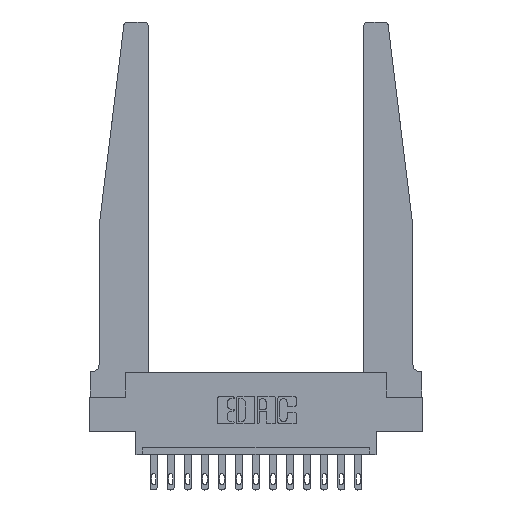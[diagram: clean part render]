
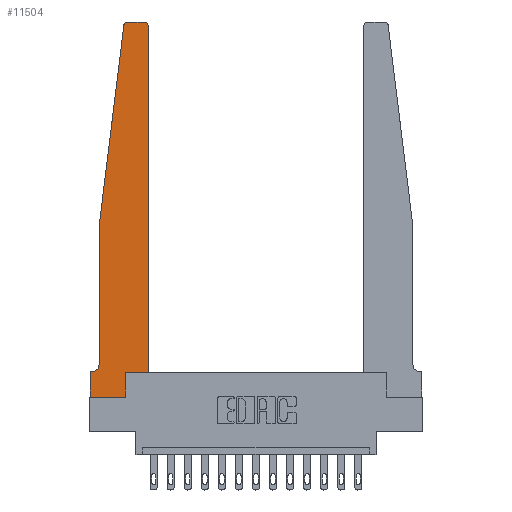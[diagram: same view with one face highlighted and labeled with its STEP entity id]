
A CAD part, top view. The second image highlights one B-rep face of the part: STEP entity #11504.
In plain terms, the highlighted planar face has unit normal (0, 0, 1).
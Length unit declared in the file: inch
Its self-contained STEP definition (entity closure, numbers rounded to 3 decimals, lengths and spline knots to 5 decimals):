
#85 = ORIENTED_EDGE ( 'NONE', *, *, #14203, .T. ) ;
#145 = AXIS2_PLACEMENT_3D ( 'NONE', #423, #7036, #6949 ) ;
#175 = CARTESIAN_POINT ( 'NONE',  ( 0.2605, 0., 0.37 ) ) ;
#423 = CARTESIAN_POINT ( 'NONE',  ( 0.395, 2.72, 0.37 ) ) ;
#473 = DIRECTION ( 'NONE',  ( -1., 0., 0. ) ) ;
#616 = AXIS2_PLACEMENT_3D ( 'NONE', #3049, #8361, #13669 ) ;
#685 = AXIS2_PLACEMENT_3D ( 'NONE', #10924, #15071, #6971 ) ;
#771 = VERTEX_POINT ( 'NONE', #175 ) ;
#1100 = CARTESIAN_POINT ( 'NONE',  ( 0., 0., 0.37 ) ) ;
#1101 = DIRECTION ( 'NONE',  ( 0., 1., 0. ) ) ;
#1122 = DIRECTION ( 'NONE',  ( 0., 0., 1. ) ) ;
#1302 = EDGE_CURVE ( 'NONE', #15732, #11408, #9125, .T. ) ;
#1695 = DIRECTION ( 'NONE',  ( 0., 1., 0. ) ) ;
#1718 = ORIENTED_EDGE ( 'NONE', *, *, #15096, .T. ) ;
#1753 = FACE_OUTER_BOUND ( 'NONE', #12169, .T. ) ;
#2190 = VERTEX_POINT ( 'NONE', #6112 ) ;
#2612 = VERTEX_POINT ( 'NONE', #16563 ) ;
#2880 = EDGE_CURVE ( 'NONE', #2612, #6151, #5559, .T. ) ;
#2933 = CIRCLE ( 'NONE', #145, 0.03 ) ;
#3001 = CARTESIAN_POINT ( 'NONE',  ( 0.24675, 2.72367, 0.37 ) ) ;
#3049 = CARTESIAN_POINT ( 'NONE',  ( 0.015, 0.2375, 0.37 ) ) ;
#3101 = VERTEX_POINT ( 'NONE', #17147 ) ;
#3812 = DIRECTION ( 'NONE',  ( 0., -1., 0. ) ) ;
#3958 = ORIENTED_EDGE ( 'NONE', *, *, #2880, .T. ) ;
#4111 = VERTEX_POINT ( 'NONE', #5738 ) ;
#4296 = EDGE_CURVE ( 'NONE', #4111, #2190, #6340, .T. ) ;
#4434 = ORIENTED_EDGE ( 'NONE', *, *, #4815, .T. ) ;
#4511 = LINE ( 'NONE', #15226, #11568 ) ;
#4791 = CARTESIAN_POINT ( 'NONE',  ( 0.065, 1.25, 0.37 ) ) ;
#4815 = EDGE_CURVE ( 'NONE', #771, #12473, #13539, .T. ) ;
#5033 = CARTESIAN_POINT ( 'NONE',  ( 0.25, 2.75, 0.37 ) ) ;
#5289 = DIRECTION ( 'NONE',  ( -1., 0., 0. ) ) ;
#5357 = VERTEX_POINT ( 'NONE', #11639 ) ;
#5559 = LINE ( 'NONE', #16190, #6957 ) ;
#5592 = ORIENTED_EDGE ( 'NONE', *, *, #10741, .T. ) ;
#5650 = ORIENTED_EDGE ( 'NONE', *, *, #10517, .T. ) ;
#5738 = CARTESIAN_POINT ( 'NONE',  ( 0.395, 2.75, 0.37 ) ) ;
#6112 = CARTESIAN_POINT ( 'NONE',  ( 0.27653, 2.75, 0.37 ) ) ;
#6151 = VERTEX_POINT ( 'NONE', #17052 ) ;
#6340 = LINE ( 'NONE', #5033, #9158 ) ;
#6438 = DIRECTION ( 'NONE',  ( 1., 0., 0. ) ) ;
#6949 = DIRECTION ( 'NONE',  ( 1., 0., 0. ) ) ;
#6957 = VECTOR ( 'NONE', #12281, 39.37008 ) ;
#6971 = DIRECTION ( 'NONE',  ( 1., 0., 0. ) ) ;
#7003 = CARTESIAN_POINT ( 'NONE',  ( 0.2605, 0.18, 0.37 ) ) ;
#7008 = VECTOR ( 'NONE', #8974, 39.37008 ) ;
#7036 = DIRECTION ( 'NONE',  ( 0., 0., 1. ) ) ;
#7101 = VECTOR ( 'NONE', #473, 39.37008 ) ;
#7243 = ORIENTED_EDGE ( 'NONE', *, *, #8832, .T. ) ;
#7322 = VECTOR ( 'NONE', #1101, 39.37008 ) ;
#7410 = CIRCLE ( 'NONE', #17164, 0.03 ) ;
#7605 = ORIENTED_EDGE ( 'NONE', *, *, #1302, .T. ) ;
#7744 = LINE ( 'NONE', #4791, #7008 ) ;
#8196 = VECTOR ( 'NONE', #3812, 39.37008 ) ;
#8361 = DIRECTION ( 'NONE',  ( 0., 0., -1. ) ) ;
#8695 = ORIENTED_EDGE ( 'NONE', *, *, #4296, .T. ) ;
#8832 = EDGE_CURVE ( 'NONE', #6151, #3101, #10650, .T. ) ;
#8894 = EDGE_CURVE ( 'NONE', #11261, #2612, #7744, .T. ) ;
#8974 = DIRECTION ( 'NONE',  ( -0.122, -0.992, 0. ) ) ;
#9125 = LINE ( 'NONE', #1100, #8196 ) ;
#9158 = VECTOR ( 'NONE', #5289, 39.37008 ) ;
#9843 = VECTOR ( 'NONE', #12177, 39.37008 ) ;
#9886 = CARTESIAN_POINT ( 'NONE',  ( 0.065, 0.1875, 0.37 ) ) ;
#10517 = EDGE_CURVE ( 'NONE', #5357, #16616, #14339, .T. ) ;
#10575 = CARTESIAN_POINT ( 'NONE',  ( 0., 0., 0.37 ) ) ;
#10650 = CIRCLE ( 'NONE', #616, 0.05 ) ;
#10741 = EDGE_CURVE ( 'NONE', #11408, #771, #13214, .T. ) ;
#10924 = CARTESIAN_POINT ( 'NONE',  ( 0., 0.1875, 0.37 ) ) ;
#11150 = CARTESIAN_POINT ( 'NONE',  ( 0.425, 2.72, 0.37 ) ) ;
#11184 = PLANE ( 'NONE',  #685 ) ;
#11261 = VERTEX_POINT ( 'NONE', #3001 ) ;
#11408 = VERTEX_POINT ( 'NONE', #10575 ) ;
#11504 = ADVANCED_FACE ( 'NONE', ( #1753 ), #11184, .T. ) ;
#11568 = VECTOR ( 'NONE', #13663, 39.37008 ) ;
#11639 = CARTESIAN_POINT ( 'NONE',  ( 0.425, 0.18, 0.37 ) ) ;
#11848 = CARTESIAN_POINT ( 'NONE',  ( 0., 0.1875, 0.37 ) ) ;
#12169 = EDGE_LOOP ( 'NONE', ( #8695, #15881, #12314, #3958, #7243, #1718, #7605, #5592, #4434, #13002, #5650, #85 ) ) ;
#12177 = DIRECTION ( 'NONE',  ( 1., 0., 0. ) ) ;
#12281 = DIRECTION ( 'NONE',  ( 0., -1., 0. ) ) ;
#12314 = ORIENTED_EDGE ( 'NONE', *, *, #8894, .T. ) ;
#12408 = LINE ( 'NONE', #9886, #7101 ) ;
#12473 = VERTEX_POINT ( 'NONE', #15520 ) ;
#13002 = ORIENTED_EDGE ( 'NONE', *, *, #14178, .T. ) ;
#13056 = CARTESIAN_POINT ( 'NONE',  ( 0.27653, 2.72, 0.37 ) ) ;
#13214 = LINE ( 'NONE', #16081, #9843 ) ;
#13539 = LINE ( 'NONE', #7003, #16159 ) ;
#13663 = DIRECTION ( 'NONE',  ( 1., 0., 0. ) ) ;
#13669 = DIRECTION ( 'NONE',  ( -1., 0., 0. ) ) ;
#14165 = CARTESIAN_POINT ( 'NONE',  ( 0.425, 0.18, 0.37 ) ) ;
#14178 = EDGE_CURVE ( 'NONE', #12473, #5357, #4511, .T. ) ;
#14203 = EDGE_CURVE ( 'NONE', #16616, #4111, #2933, .T. ) ;
#14339 = LINE ( 'NONE', #14165, #7322 ) ;
#15071 = DIRECTION ( 'NONE',  ( 0., 0., 1. ) ) ;
#15096 = EDGE_CURVE ( 'NONE', #3101, #15732, #12408, .T. ) ;
#15226 = CARTESIAN_POINT ( 'NONE',  ( 0.425, 0.18, 0.37 ) ) ;
#15520 = CARTESIAN_POINT ( 'NONE',  ( 0.2605, 0.18, 0.37 ) ) ;
#15732 = VERTEX_POINT ( 'NONE', #11848 ) ;
#15881 = ORIENTED_EDGE ( 'NONE', *, *, #16460, .T. ) ;
#16081 = CARTESIAN_POINT ( 'NONE',  ( 0., 0., 0.37 ) ) ;
#16159 = VECTOR ( 'NONE', #1695, 39.37008 ) ;
#16190 = CARTESIAN_POINT ( 'NONE',  ( 0.065, 1.25, 0.37 ) ) ;
#16460 = EDGE_CURVE ( 'NONE', #2190, #11261, #7410, .T. ) ;
#16563 = CARTESIAN_POINT ( 'NONE',  ( 0.065, 1.25, 0.37 ) ) ;
#16616 = VERTEX_POINT ( 'NONE', #11150 ) ;
#17052 = CARTESIAN_POINT ( 'NONE',  ( 0.065, 0.2375, 0.37 ) ) ;
#17147 = CARTESIAN_POINT ( 'NONE',  ( 0.015, 0.1875, 0.37 ) ) ;
#17164 = AXIS2_PLACEMENT_3D ( 'NONE', #13056, #1122, #6438 ) ;
